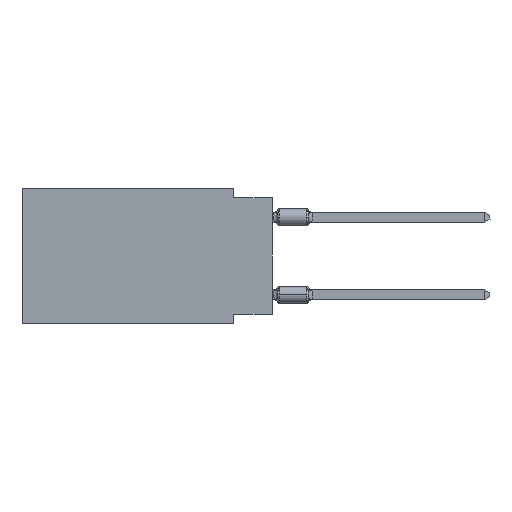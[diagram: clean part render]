
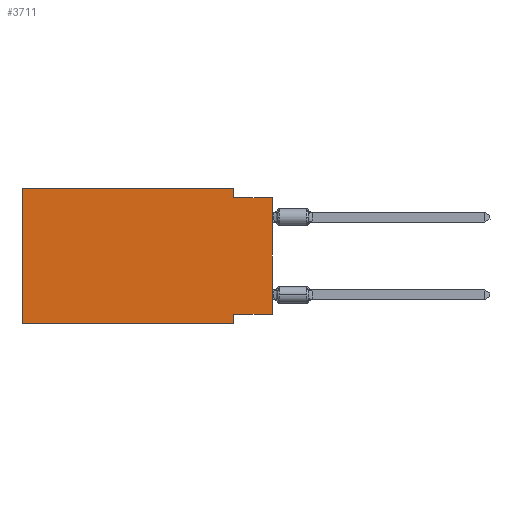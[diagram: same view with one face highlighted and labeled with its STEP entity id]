
A CAD part, left-side view. The second image highlights one B-rep face of the part: STEP entity #3711.
In plain terms, the highlighted planar face has unit normal (-1, 0, 0).
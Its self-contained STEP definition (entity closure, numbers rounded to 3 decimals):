
#105 = DIRECTION ( 'NONE',  ( 0., 0., -1. ) ) ;
#229 = CARTESIAN_POINT ( 'NONE',  ( 0., 2.54, -0.635 ) ) ;
#415 = ORIENTED_EDGE ( 'NONE', *, *, #10662, .F. ) ;
#506 = VECTOR ( 'NONE', #11736, 1000. ) ;
#1135 = VECTOR ( 'NONE', #2588, 1000. ) ;
#1250 = LINE ( 'NONE', #5876, #5188 ) ;
#1267 = CARTESIAN_POINT ( 'NONE',  ( 0., 2.54, 0. ) ) ;
#1516 = ORIENTED_EDGE ( 'NONE', *, *, #14778, .T. ) ;
#1605 = VECTOR ( 'NONE', #12346, 1000. ) ;
#1754 = EDGE_CURVE ( 'NONE', #7157, #7641, #9565, .T. ) ;
#1800 = VERTEX_POINT ( 'NONE', #8571 ) ;
#2588 = DIRECTION ( 'NONE',  ( 0., 0., 1. ) ) ;
#2771 = DIRECTION ( 'NONE',  ( 1., 0., 0. ) ) ;
#2855 = LINE ( 'NONE', #3771, #6324 ) ;
#2880 = VERTEX_POINT ( 'NONE', #14315 ) ;
#3569 = ORIENTED_EDGE ( 'NONE', *, *, #3680, .F. ) ;
#3636 = VERTEX_POINT ( 'NONE', #8024 ) ;
#3680 = EDGE_CURVE ( 'NONE', #9673, #7946, #12742, .T. ) ;
#3711 = ADVANCED_FACE ( 'NONE', ( #13190 ), #8322, .F. ) ;
#3771 = CARTESIAN_POINT ( 'NONE',  ( 0., 16.383, 0. ) ) ;
#4053 = CARTESIAN_POINT ( 'NONE',  ( 0., 0., -8.255 ) ) ;
#4155 = AXIS2_PLACEMENT_3D ( 'NONE', #12110, #2771, #14334 ) ;
#4219 = LINE ( 'NONE', #7712, #1605 ) ;
#4271 = DIRECTION ( 'NONE',  ( 0., -1., 0. ) ) ;
#4347 = CARTESIAN_POINT ( 'NONE',  ( 0., 2.54, 0. ) ) ;
#4467 = CARTESIAN_POINT ( 'NONE',  ( 0., 0., -0.635 ) ) ;
#5188 = VECTOR ( 'NONE', #105, 1000. ) ;
#5245 = CARTESIAN_POINT ( 'NONE',  ( 0., 0., -0.635 ) ) ;
#5876 = CARTESIAN_POINT ( 'NONE',  ( 0., 2.54, -8.89 ) ) ;
#5938 = VECTOR ( 'NONE', #4271, 1000. ) ;
#6324 = VECTOR ( 'NONE', #10830, 1000. ) ;
#6368 = CARTESIAN_POINT ( 'NONE',  ( 0., 0., 0. ) ) ;
#6544 = LINE ( 'NONE', #13542, #5938 ) ;
#6686 = EDGE_CURVE ( 'NONE', #8431, #9673, #2855, .T. ) ;
#7157 = VERTEX_POINT ( 'NONE', #4053 ) ;
#7641 = VERTEX_POINT ( 'NONE', #5245 ) ;
#7712 = CARTESIAN_POINT ( 'NONE',  ( 0., 16.383, 0. ) ) ;
#7946 = VERTEX_POINT ( 'NONE', #229 ) ;
#8024 = CARTESIAN_POINT ( 'NONE',  ( 0., 2.54, -8.89 ) ) ;
#8322 = PLANE ( 'NONE',  #4155 ) ;
#8431 = VERTEX_POINT ( 'NONE', #11670 ) ;
#8457 = ORIENTED_EDGE ( 'NONE', *, *, #6686, .F. ) ;
#8571 = CARTESIAN_POINT ( 'NONE',  ( 0., 2.54, -8.255 ) ) ;
#8839 = VECTOR ( 'NONE', #13743, 1000. ) ;
#9346 = EDGE_CURVE ( 'NONE', #7157, #1800, #9462, .T. ) ;
#9462 = LINE ( 'NONE', #13898, #12216 ) ;
#9565 = LINE ( 'NONE', #6368, #1135 ) ;
#9673 = VERTEX_POINT ( 'NONE', #4347 ) ;
#10376 = ORIENTED_EDGE ( 'NONE', *, *, #1754, .T. ) ;
#10662 = EDGE_CURVE ( 'NONE', #7946, #7641, #13897, .T. ) ;
#10830 = DIRECTION ( 'NONE',  ( 0., -1., 0. ) ) ;
#11072 = EDGE_LOOP ( 'NONE', ( #10376, #415, #3569, #8457, #14883, #1516, #12630, #14477 ) ) ;
#11670 = CARTESIAN_POINT ( 'NONE',  ( 0., 16.383, 0. ) ) ;
#11736 = DIRECTION ( 'NONE',  ( 0., 0., -1. ) ) ;
#12110 = CARTESIAN_POINT ( 'NONE',  ( 0., 16.383, 0. ) ) ;
#12155 = EDGE_CURVE ( 'NONE', #2880, #8431, #4219, .T. ) ;
#12216 = VECTOR ( 'NONE', #12665, 1000. ) ;
#12346 = DIRECTION ( 'NONE',  ( 0., 0., 1. ) ) ;
#12630 = ORIENTED_EDGE ( 'NONE', *, *, #14593, .F. ) ;
#12665 = DIRECTION ( 'NONE',  ( 0., 1., 0. ) ) ;
#12742 = LINE ( 'NONE', #1267, #506 ) ;
#13190 = FACE_OUTER_BOUND ( 'NONE', #11072, .T. ) ;
#13542 = CARTESIAN_POINT ( 'NONE',  ( 0., 16.383, -8.89 ) ) ;
#13743 = DIRECTION ( 'NONE',  ( 0., -1., 0. ) ) ;
#13897 = LINE ( 'NONE', #4467, #8839 ) ;
#13898 = CARTESIAN_POINT ( 'NONE',  ( 0., 0., -8.255 ) ) ;
#14315 = CARTESIAN_POINT ( 'NONE',  ( 0., 16.383, -8.89 ) ) ;
#14334 = DIRECTION ( 'NONE',  ( 0., 0., -1. ) ) ;
#14477 = ORIENTED_EDGE ( 'NONE', *, *, #9346, .F. ) ;
#14593 = EDGE_CURVE ( 'NONE', #1800, #3636, #1250, .T. ) ;
#14778 = EDGE_CURVE ( 'NONE', #2880, #3636, #6544, .T. ) ;
#14883 = ORIENTED_EDGE ( 'NONE', *, *, #12155, .F. ) ;
